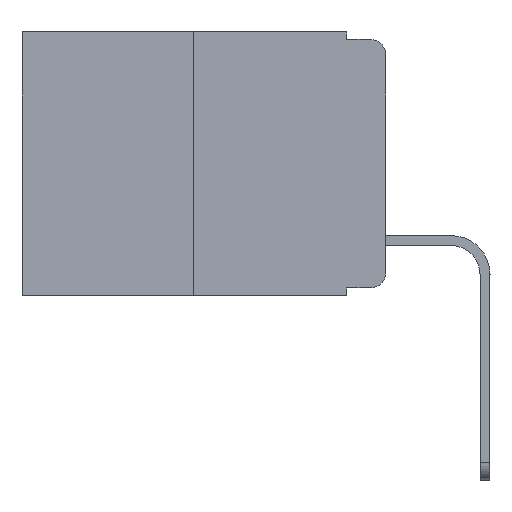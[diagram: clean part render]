
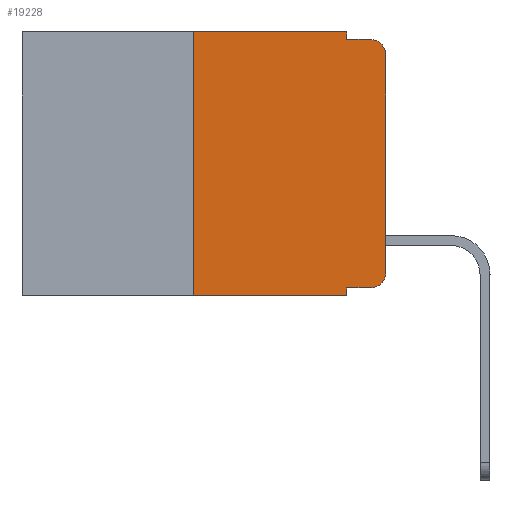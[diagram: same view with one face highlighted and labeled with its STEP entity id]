
A CAD part, left-side view. The second image highlights one B-rep face of the part: STEP entity #19228.
In plain terms, the highlighted planar face has unit normal (-1, 0, 0).
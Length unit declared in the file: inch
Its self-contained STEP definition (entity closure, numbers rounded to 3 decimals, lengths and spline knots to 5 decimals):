
#331 = CARTESIAN_POINT ( 'NONE',  ( 0., 0.051, -0.01 ) ) ;
#758 = VERTEX_POINT ( 'NONE', #11931 ) ;
#818 = CARTESIAN_POINT ( 'NONE',  ( 0., 0.473, -0.343 ) ) ;
#980 = VERTEX_POINT ( 'NONE', #5749 ) ;
#1229 = VERTEX_POINT ( 'NONE', #13918 ) ;
#1317 = VERTEX_POINT ( 'NONE', #15701 ) ;
#1939 = DIRECTION ( 'NONE',  ( 0., 0., -1. ) ) ;
#2222 = ORIENTED_EDGE ( 'NONE', *, *, #18496, .F. ) ;
#2255 = LINE ( 'NONE', #20947, #7586 ) ;
#2375 = ORIENTED_EDGE ( 'NONE', *, *, #21281, .T. ) ;
#2465 = CARTESIAN_POINT ( 'NONE',  ( 0., 0., 0. ) ) ;
#2614 = DIRECTION ( 'NONE',  ( 0., 0., -1. ) ) ;
#2632 = AXIS2_PLACEMENT_3D ( 'NONE', #14112, #5963, #2614 ) ;
#3346 = EDGE_CURVE ( 'NONE', #1229, #758, #19269, .T. ) ;
#3514 = VERTEX_POINT ( 'NONE', #15245 ) ;
#3541 = EDGE_CURVE ( 'NONE', #3514, #14517, #4230, .T. ) ;
#3565 = LINE ( 'NONE', #8649, #18319 ) ;
#3919 = CARTESIAN_POINT ( 'NONE',  ( 0., 0.02, -0.313 ) ) ;
#4230 = CIRCLE ( 'NONE', #2632, 0.02 ) ;
#4396 = CARTESIAN_POINT ( 'NONE',  ( 0., 0.25, -0.343 ) ) ;
#5326 = VERTEX_POINT ( 'NONE', #331 ) ;
#5406 = VERTEX_POINT ( 'NONE', #4396 ) ;
#5749 = CARTESIAN_POINT ( 'NONE',  ( 0., 0.051, 0. ) ) ;
#5895 = LINE ( 'NONE', #21261, #15074 ) ;
#5928 = EDGE_CURVE ( 'NONE', #15407, #16845, #19445, .T. ) ;
#5963 = DIRECTION ( 'NONE',  ( -1., 0., 0. ) ) ;
#5992 = AXIS2_PLACEMENT_3D ( 'NONE', #10288, #8681, #1939 ) ;
#6253 = VECTOR ( 'NONE', #18781, 39.37008 ) ;
#6586 = ORIENTED_EDGE ( 'NONE', *, *, #20235, .F. ) ;
#7201 = LINE ( 'NONE', #2465, #19842 ) ;
#7581 = ORIENTED_EDGE ( 'NONE', *, *, #3346, .F. ) ;
#7586 = VECTOR ( 'NONE', #20665, 39.37008 ) ;
#8539 = DIRECTION ( 'NONE',  ( 0., 0., -1. ) ) ;
#8649 = CARTESIAN_POINT ( 'NONE',  ( 0., 0.473, 0. ) ) ;
#8681 = DIRECTION ( 'NONE',  ( 1., 0., 0. ) ) ;
#8827 = FACE_OUTER_BOUND ( 'NONE', #9852, .T. ) ;
#9030 = DIRECTION ( 'NONE',  ( 0., 0., -1. ) ) ;
#9727 = ORIENTED_EDGE ( 'NONE', *, *, #3541, .T. ) ;
#9781 = VECTOR ( 'NONE', #8539, 39.37008 ) ;
#9852 = EDGE_LOOP ( 'NONE', ( #2375, #9727, #2222, #10078, #17795, #6586, #17343, #7581, #9948, #12881 ) ) ;
#9948 = ORIENTED_EDGE ( 'NONE', *, *, #11691, .T. ) ;
#10078 = ORIENTED_EDGE ( 'NONE', *, *, #21845, .F. ) ;
#10258 = DIRECTION ( 'NONE',  ( 0., -1., 0. ) ) ;
#10288 = CARTESIAN_POINT ( 'NONE',  ( 0., 0.473, 0. ) ) ;
#10397 = CARTESIAN_POINT ( 'NONE',  ( 0., 0.051, -0.01 ) ) ;
#11461 = EDGE_CURVE ( 'NONE', #1317, #980, #3565, .T. ) ;
#11691 = EDGE_CURVE ( 'NONE', #1229, #15407, #2255, .T. ) ;
#11931 = CARTESIAN_POINT ( 'NONE',  ( 0., 0.051, -0.343 ) ) ;
#12549 = CARTESIAN_POINT ( 'NONE',  ( 0., 0.051, 0. ) ) ;
#12881 = ORIENTED_EDGE ( 'NONE', *, *, #5928, .T. ) ;
#13164 = EDGE_CURVE ( 'NONE', #5406, #758, #17990, .T. ) ;
#13897 = CARTESIAN_POINT ( 'NONE',  ( 0., 0., -0.313 ) ) ;
#13918 = CARTESIAN_POINT ( 'NONE',  ( 0., 0.051, -0.333 ) ) ;
#14112 = CARTESIAN_POINT ( 'NONE',  ( 0., 0.02, -0.03 ) ) ;
#14148 = DIRECTION ( 'NONE',  ( 0., 0., -1. ) ) ;
#14368 = DIRECTION ( 'NONE',  ( 0., 0., 1. ) ) ;
#14517 = VERTEX_POINT ( 'NONE', #20329 ) ;
#15074 = VECTOR ( 'NONE', #14368, 39.37008 ) ;
#15245 = CARTESIAN_POINT ( 'NONE',  ( 0., 0., -0.03 ) ) ;
#15407 = VERTEX_POINT ( 'NONE', #15704 ) ;
#15426 = CARTESIAN_POINT ( 'NONE',  ( 0., 0.051, 0. ) ) ;
#15701 = CARTESIAN_POINT ( 'NONE',  ( 0., 0.25, 0. ) ) ;
#15704 = CARTESIAN_POINT ( 'NONE',  ( 0., 0.02, -0.333 ) ) ;
#15714 = LINE ( 'NONE', #10397, #6253 ) ;
#16845 = VERTEX_POINT ( 'NONE', #13897 ) ;
#17343 = ORIENTED_EDGE ( 'NONE', *, *, #13164, .T. ) ;
#17795 = ORIENTED_EDGE ( 'NONE', *, *, #11461, .F. ) ;
#17990 = LINE ( 'NONE', #818, #18517 ) ;
#18319 = VECTOR ( 'NONE', #10258, 39.37008 ) ;
#18496 = EDGE_CURVE ( 'NONE', #5326, #14517, #15714, .T. ) ;
#18517 = VECTOR ( 'NONE', #19790, 39.37008 ) ;
#18781 = DIRECTION ( 'NONE',  ( 0., -1., 0. ) ) ;
#19018 = LINE ( 'NONE', #12549, #21431 ) ;
#19113 = DIRECTION ( 'NONE',  ( -1., 0., 0. ) ) ;
#19228 = ADVANCED_FACE ( 'NONE', ( #8827 ), #20321, .F. ) ;
#19269 = LINE ( 'NONE', #15426, #9781 ) ;
#19445 = CIRCLE ( 'NONE', #21208, 0.02 ) ;
#19790 = DIRECTION ( 'NONE',  ( 0., -1., 0. ) ) ;
#19842 = VECTOR ( 'NONE', #20838, 39.37008 ) ;
#20235 = EDGE_CURVE ( 'NONE', #5406, #1317, #5895, .T. ) ;
#20321 = PLANE ( 'NONE',  #5992 ) ;
#20329 = CARTESIAN_POINT ( 'NONE',  ( 0., 0.02, -0.01 ) ) ;
#20665 = DIRECTION ( 'NONE',  ( 0., -1., 0. ) ) ;
#20838 = DIRECTION ( 'NONE',  ( 0., 0., 1. ) ) ;
#20947 = CARTESIAN_POINT ( 'NONE',  ( 0., 0.051, -0.333 ) ) ;
#21208 = AXIS2_PLACEMENT_3D ( 'NONE', #3919, #19113, #9030 ) ;
#21261 = CARTESIAN_POINT ( 'NONE',  ( 0., 0.25, 0. ) ) ;
#21281 = EDGE_CURVE ( 'NONE', #16845, #3514, #7201, .T. ) ;
#21431 = VECTOR ( 'NONE', #14148, 39.37008 ) ;
#21845 = EDGE_CURVE ( 'NONE', #980, #5326, #19018, .T. ) ;
